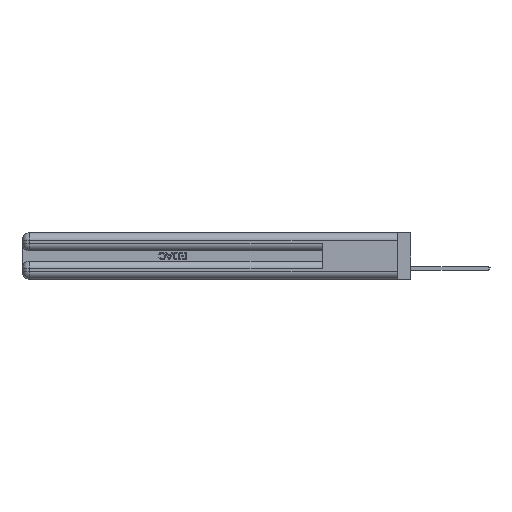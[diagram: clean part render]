
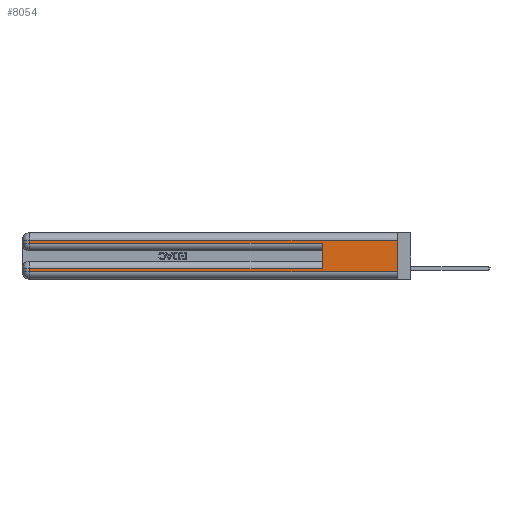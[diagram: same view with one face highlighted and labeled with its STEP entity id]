
A CAD part, left-side view. The second image highlights one B-rep face of the part: STEP entity #8054.
In plain terms, the highlighted planar face has unit normal (-1, 0, 0).
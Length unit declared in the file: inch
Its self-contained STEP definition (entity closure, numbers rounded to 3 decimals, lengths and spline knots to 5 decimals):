
#1663 = ORIENTED_EDGE ( 'NONE', *, *, #44219, .T. ) ;
#2050 = LINE ( 'NONE', #8533, #25195 ) ;
#2306 = EDGE_CURVE ( 'NONE', #16997, #41839, #22376, .T. ) ;
#2520 = CARTESIAN_POINT ( 'NONE',  ( 0., 0., 0.06 ) ) ;
#2853 = DIRECTION ( 'NONE',  ( 0., 0., -1. ) ) ;
#3279 = EDGE_CURVE ( 'NONE', #18537, #27374, #27904, .T. ) ;
#3619 = VECTOR ( 'NONE', #41370, 39.37008 ) ;
#4630 = VECTOR ( 'NONE', #44683, 39.37008 ) ;
#5786 = EDGE_CURVE ( 'NONE', #8416, #40994, #33775, .T. ) ;
#6711 = ORIENTED_EDGE ( 'NONE', *, *, #3279, .T. ) ;
#8054 = ADVANCED_FACE ( 'NONE', ( #9964 ), #32851, .F. ) ;
#8416 = VERTEX_POINT ( 'NONE', #43489 ) ;
#8533 = CARTESIAN_POINT ( 'NONE',  ( 0., 0., 0.31 ) ) ;
#8847 = CARTESIAN_POINT ( 'NONE',  ( 0., 0., 0.285 ) ) ;
#9150 = DIRECTION ( 'NONE',  ( 0., -1., 0. ) ) ;
#9964 = FACE_OUTER_BOUND ( 'NONE', #30633, .T. ) ;
#11335 = LINE ( 'NONE', #2520, #37130 ) ;
#15541 = ORIENTED_EDGE ( 'NONE', *, *, #26473, .T. ) ;
#16997 = VERTEX_POINT ( 'NONE', #43053 ) ;
#17365 = CARTESIAN_POINT ( 'NONE',  ( 0., 2.94, 0.06 ) ) ;
#17980 = CARTESIAN_POINT ( 'NONE',  ( 0., 0., 0.06 ) ) ;
#18537 = VERTEX_POINT ( 'NONE', #29445 ) ;
#18988 = CARTESIAN_POINT ( 'NONE',  ( 0., 0.6, 0.145 ) ) ;
#19071 = ORIENTED_EDGE ( 'NONE', *, *, #5786, .T. ) ;
#19129 = ORIENTED_EDGE ( 'NONE', *, *, #2306, .F. ) ;
#19609 = EDGE_CURVE ( 'NONE', #16997, #38606, #2050, .T. ) ;
#19640 = DIRECTION ( 'NONE',  ( 0., 1., 0. ) ) ;
#20357 = LINE ( 'NONE', #37722, #26340 ) ;
#20590 = CARTESIAN_POINT ( 'NONE',  ( 0., 2.94, 0.31 ) ) ;
#20962 = ORIENTED_EDGE ( 'NONE', *, *, #41533, .F. ) ;
#22376 = LINE ( 'NONE', #30721, #3619 ) ;
#22566 = CARTESIAN_POINT ( 'NONE',  ( 0., 0.6, 0.285 ) ) ;
#22733 = EDGE_CURVE ( 'NONE', #40787, #41839, #11335, .T. ) ;
#23940 = VECTOR ( 'NONE', #30316, 39.37008 ) ;
#24693 = ORIENTED_EDGE ( 'NONE', *, *, #22733, .T. ) ;
#25195 = VECTOR ( 'NONE', #19640, 39.37008 ) ;
#26260 = LINE ( 'NONE', #18988, #36719 ) ;
#26340 = VECTOR ( 'NONE', #2853, 39.37008 ) ;
#26473 = EDGE_CURVE ( 'NONE', #38606, #8416, #20357, .T. ) ;
#26626 = ORIENTED_EDGE ( 'NONE', *, *, #19609, .T. ) ;
#27374 = VERTEX_POINT ( 'NONE', #35516 ) ;
#27716 = LINE ( 'NONE', #41315, #4630 ) ;
#27904 = LINE ( 'NONE', #35634, #37266 ) ;
#29402 = DIRECTION ( 'NONE',  ( 0., 0., -1. ) ) ;
#29445 = CARTESIAN_POINT ( 'NONE',  ( 0., 0.6, 0.085 ) ) ;
#29829 = DIRECTION ( 'NONE',  ( 0., 0., 1. ) ) ;
#30316 = DIRECTION ( 'NONE',  ( 0., -1., 0. ) ) ;
#30633 = EDGE_LOOP ( 'NONE', ( #19129, #26626, #15541, #19071, #20962, #6711, #1663, #24693 ) ) ;
#30721 = CARTESIAN_POINT ( 'NONE',  ( 0., 0., 0.37 ) ) ;
#32851 = PLANE ( 'NONE',  #42211 ) ;
#33775 = LINE ( 'NONE', #8847, #23940 ) ;
#35516 = CARTESIAN_POINT ( 'NONE',  ( 0., 2.94, 0.085 ) ) ;
#35634 = CARTESIAN_POINT ( 'NONE',  ( 0., 0., 0.085 ) ) ;
#36719 = VECTOR ( 'NONE', #29829, 39.37008 ) ;
#36987 = DIRECTION ( 'NONE',  ( 0., 1., 0. ) ) ;
#37130 = VECTOR ( 'NONE', #9150, 39.37008 ) ;
#37266 = VECTOR ( 'NONE', #36987, 39.37008 ) ;
#37722 = CARTESIAN_POINT ( 'NONE',  ( 0., 2.94, 0.37 ) ) ;
#38606 = VERTEX_POINT ( 'NONE', #20590 ) ;
#38690 = DIRECTION ( 'NONE',  ( 1., 0., 0. ) ) ;
#40787 = VERTEX_POINT ( 'NONE', #17365 ) ;
#40994 = VERTEX_POINT ( 'NONE', #22566 ) ;
#41315 = CARTESIAN_POINT ( 'NONE',  ( 0., 2.94, 0.37 ) ) ;
#41370 = DIRECTION ( 'NONE',  ( 0., 0., -1. ) ) ;
#41533 = EDGE_CURVE ( 'NONE', #18537, #40994, #26260, .T. ) ;
#41839 = VERTEX_POINT ( 'NONE', #17980 ) ;
#42211 = AXIS2_PLACEMENT_3D ( 'NONE', #42902, #38690, #29402 ) ;
#42902 = CARTESIAN_POINT ( 'NONE',  ( 0., 0., 0.37 ) ) ;
#43053 = CARTESIAN_POINT ( 'NONE',  ( 0., 0., 0.31 ) ) ;
#43489 = CARTESIAN_POINT ( 'NONE',  ( 0., 2.94, 0.285 ) ) ;
#44219 = EDGE_CURVE ( 'NONE', #27374, #40787, #27716, .T. ) ;
#44683 = DIRECTION ( 'NONE',  ( 0., 0., -1. ) ) ;
